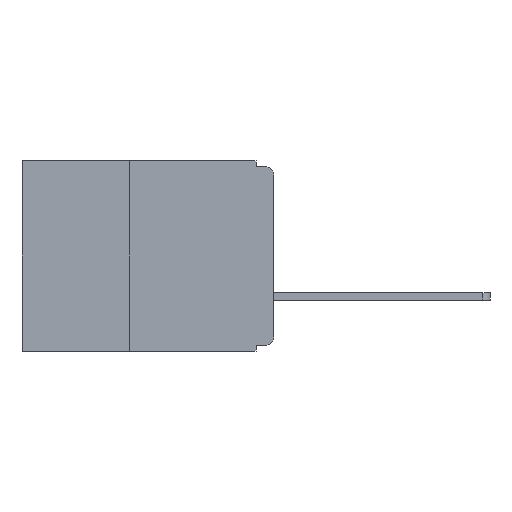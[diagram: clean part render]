
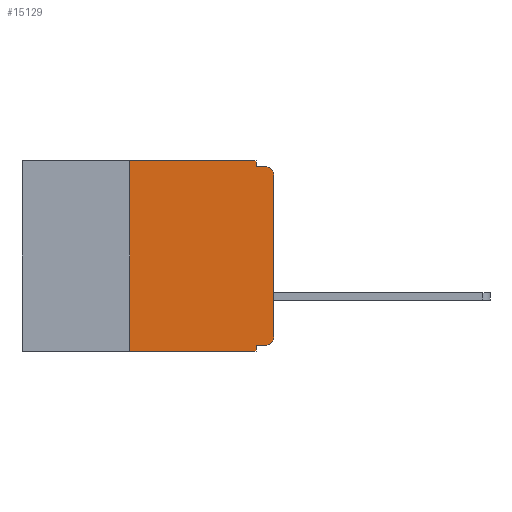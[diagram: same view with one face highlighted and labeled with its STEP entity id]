
A CAD part, left-side view. The second image highlights one B-rep face of the part: STEP entity #15129.
In plain terms, the highlighted planar face has unit normal (-1, 0, 0).
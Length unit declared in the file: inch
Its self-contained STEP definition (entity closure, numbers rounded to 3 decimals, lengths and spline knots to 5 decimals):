
#143 = VECTOR ( 'NONE', #6150, 39.37008 ) ;
#195 = VERTEX_POINT ( 'NONE', #9062 ) ;
#268 = DIRECTION ( 'NONE',  ( 0., -1., 0. ) ) ;
#573 = EDGE_CURVE ( 'NONE', #13013, #2886, #6966, .T. ) ;
#949 = CARTESIAN_POINT ( 'NONE',  ( 0., 0., -0.025 ) ) ;
#1029 = AXIS2_PLACEMENT_3D ( 'NONE', #12722, #14806, #8148 ) ;
#1222 = LINE ( 'NONE', #7967, #4286 ) ;
#1225 = ORIENTED_EDGE ( 'NONE', *, *, #9158, .F. ) ;
#1617 = DIRECTION ( 'NONE',  ( 0., 0., 1. ) ) ;
#1634 = DIRECTION ( 'NONE',  ( 0., 0., -1. ) ) ;
#1780 = CARTESIAN_POINT ( 'NONE',  ( 0., 0.25, -0.33 ) ) ;
#2088 = LINE ( 'NONE', #9513, #8458 ) ;
#2183 = EDGE_CURVE ( 'NONE', #5055, #10771, #7696, .T. ) ;
#2765 = DIRECTION ( 'NONE',  ( 0., 0., -1. ) ) ;
#2773 = DIRECTION ( 'NONE',  ( 0., 0., -1. ) ) ;
#2847 = DIRECTION ( 'NONE',  ( -1., 0., 0. ) ) ;
#2851 = CARTESIAN_POINT ( 'NONE',  ( 0., 0.015, -0.305 ) ) ;
#2861 = DIRECTION ( 'NONE',  ( -1., 0., 0. ) ) ;
#2886 = VERTEX_POINT ( 'NONE', #949 ) ;
#3057 = CARTESIAN_POINT ( 'NONE',  ( 0., 0.015, -0.32 ) ) ;
#3064 = ORIENTED_EDGE ( 'NONE', *, *, #14810, .F. ) ;
#3188 = VECTOR ( 'NONE', #6242, 39.37008 ) ;
#3395 = EDGE_CURVE ( 'NONE', #12024, #3842, #2088, .T. ) ;
#3477 = VERTEX_POINT ( 'NONE', #8139 ) ;
#3606 = LINE ( 'NONE', #6299, #3188 ) ;
#3687 = ORIENTED_EDGE ( 'NONE', *, *, #3395, .F. ) ;
#3842 = VERTEX_POINT ( 'NONE', #15106 ) ;
#3969 = EDGE_CURVE ( 'NONE', #2886, #10771, #15164, .T. ) ;
#4286 = VECTOR ( 'NONE', #1634, 39.37008 ) ;
#4747 = CARTESIAN_POINT ( 'NONE',  ( 0., 0.437, -0.33 ) ) ;
#5038 = VERTEX_POINT ( 'NONE', #8868 ) ;
#5055 = VERTEX_POINT ( 'NONE', #6268 ) ;
#5240 = VECTOR ( 'NONE', #1617, 39.37008 ) ;
#5291 = ORIENTED_EDGE ( 'NONE', *, *, #2183, .F. ) ;
#5355 = EDGE_CURVE ( 'NONE', #12024, #13013, #6837, .T. ) ;
#5689 = ORIENTED_EDGE ( 'NONE', *, *, #5355, .T. ) ;
#5745 = VECTOR ( 'NONE', #8526, 39.37008 ) ;
#6123 = EDGE_CURVE ( 'NONE', #195, #14283, #8539, .T. ) ;
#6150 = DIRECTION ( 'NONE',  ( 0., 0., 1. ) ) ;
#6242 = DIRECTION ( 'NONE',  ( 0., 0., -1. ) ) ;
#6268 = CARTESIAN_POINT ( 'NONE',  ( 0., 0.031, -0.01 ) ) ;
#6299 = CARTESIAN_POINT ( 'NONE',  ( 0., 0.031, 0. ) ) ;
#6400 = CARTESIAN_POINT ( 'NONE',  ( 0., 0., 0. ) ) ;
#6553 = CARTESIAN_POINT ( 'NONE',  ( 0., 0.437, 0. ) ) ;
#6837 = CIRCLE ( 'NONE', #9508, 0.015 ) ;
#6966 = LINE ( 'NONE', #6400, #143 ) ;
#7493 = EDGE_CURVE ( 'NONE', #195, #3477, #9063, .T. ) ;
#7696 = LINE ( 'NONE', #8907, #10500 ) ;
#7808 = DIRECTION ( 'NONE',  ( 0., -1., 0. ) ) ;
#7967 = CARTESIAN_POINT ( 'NONE',  ( 0., 0.031, -0.33 ) ) ;
#8139 = CARTESIAN_POINT ( 'NONE',  ( 0., 0.031, -0.33 ) ) ;
#8148 = DIRECTION ( 'NONE',  ( 0., 0., -1. ) ) ;
#8458 = VECTOR ( 'NONE', #14545, 39.37008 ) ;
#8526 = DIRECTION ( 'NONE',  ( 0., -1., 0. ) ) ;
#8539 = LINE ( 'NONE', #1780, #5240 ) ;
#8868 = CARTESIAN_POINT ( 'NONE',  ( 0., 0.031, 0. ) ) ;
#8907 = CARTESIAN_POINT ( 'NONE',  ( 0., 0., -0.01 ) ) ;
#8947 = ORIENTED_EDGE ( 'NONE', *, *, #3969, .T. ) ;
#9062 = CARTESIAN_POINT ( 'NONE',  ( 0., 0.25, -0.33 ) ) ;
#9063 = LINE ( 'NONE', #4747, #5745 ) ;
#9158 = EDGE_CURVE ( 'NONE', #14283, #5038, #11786, .T. ) ;
#9508 = AXIS2_PLACEMENT_3D ( 'NONE', #2851, #2847, #2773 ) ;
#9513 = CARTESIAN_POINT ( 'NONE',  ( 0., 0., -0.32 ) ) ;
#9902 = ORIENTED_EDGE ( 'NONE', *, *, #11927, .F. ) ;
#10001 = CARTESIAN_POINT ( 'NONE',  ( 0., 0.015, -0.01 ) ) ;
#10403 = FACE_OUTER_BOUND ( 'NONE', #11135, .T. ) ;
#10500 = VECTOR ( 'NONE', #268, 39.37008 ) ;
#10771 = VERTEX_POINT ( 'NONE', #10001 ) ;
#11115 = ORIENTED_EDGE ( 'NONE', *, *, #573, .T. ) ;
#11135 = EDGE_LOOP ( 'NONE', ( #11115, #8947, #5291, #3064, #1225, #11178, #12222, #9902, #3687, #5689 ) ) ;
#11178 = ORIENTED_EDGE ( 'NONE', *, *, #6123, .F. ) ;
#11634 = PLANE ( 'NONE',  #1029 ) ;
#11786 = LINE ( 'NONE', #6553, #14609 ) ;
#11851 = CARTESIAN_POINT ( 'NONE',  ( 0., 0., -0.305 ) ) ;
#11927 = EDGE_CURVE ( 'NONE', #3842, #3477, #1222, .T. ) ;
#12024 = VERTEX_POINT ( 'NONE', #3057 ) ;
#12222 = ORIENTED_EDGE ( 'NONE', *, *, #7493, .T. ) ;
#12722 = CARTESIAN_POINT ( 'NONE',  ( 0., 0.437, 0. ) ) ;
#13013 = VERTEX_POINT ( 'NONE', #11851 ) ;
#13822 = CARTESIAN_POINT ( 'NONE',  ( 0., 0.015, -0.025 ) ) ;
#14283 = VERTEX_POINT ( 'NONE', #14653 ) ;
#14545 = DIRECTION ( 'NONE',  ( 0., 1., 0. ) ) ;
#14609 = VECTOR ( 'NONE', #7808, 39.37008 ) ;
#14653 = CARTESIAN_POINT ( 'NONE',  ( 0., 0.25, 0. ) ) ;
#14806 = DIRECTION ( 'NONE',  ( 1., 0., 0. ) ) ;
#14810 = EDGE_CURVE ( 'NONE', #5038, #5055, #3606, .T. ) ;
#15069 = AXIS2_PLACEMENT_3D ( 'NONE', #13822, #2861, #2765 ) ;
#15106 = CARTESIAN_POINT ( 'NONE',  ( 0., 0.031, -0.32 ) ) ;
#15129 = ADVANCED_FACE ( 'NONE', ( #10403 ), #11634, .F. ) ;
#15164 = CIRCLE ( 'NONE', #15069, 0.015 ) ;
